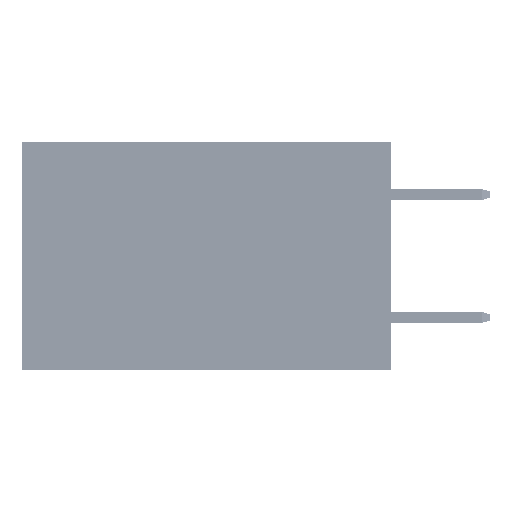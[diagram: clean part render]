
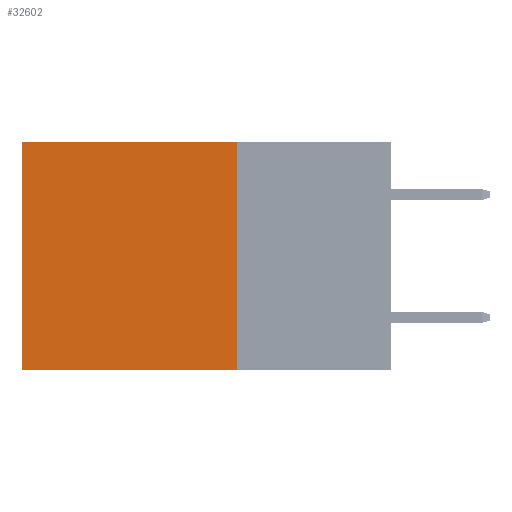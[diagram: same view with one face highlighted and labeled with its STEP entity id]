
A CAD part, left-side view. The second image highlights one B-rep face of the part: STEP entity #32602.
In plain terms, the highlighted planar face has unit normal (-1, 0, 0).
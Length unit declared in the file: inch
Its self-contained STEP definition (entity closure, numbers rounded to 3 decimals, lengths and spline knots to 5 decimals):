
#63 = DIRECTION ( 'NONE',  ( 0., 1., 0. ) ) ;
#660 = LINE ( 'NONE', #8507, #33065 ) ;
#1041 = CARTESIAN_POINT ( 'NONE',  ( 0.2875, 0.25, 0. ) ) ;
#6614 = LINE ( 'NONE', #29892, #17607 ) ;
#6809 = DIRECTION ( 'NONE',  ( 0., 0., -1. ) ) ;
#6989 = FACE_OUTER_BOUND ( 'NONE', #10618, .T. ) ;
#7064 = CARTESIAN_POINT ( 'NONE',  ( 0.2875, 0.6, 0. ) ) ;
#7995 = ORIENTED_EDGE ( 'NONE', *, *, #26236, .F. ) ;
#8343 = DIRECTION ( 'NONE',  ( 0., 0., -1. ) ) ;
#8507 = CARTESIAN_POINT ( 'NONE',  ( 0.2875, 0.25, 0. ) ) ;
#8690 = VECTOR ( 'NONE', #63, 39.37008 ) ;
#10618 = EDGE_LOOP ( 'NONE', ( #33164, #28526, #7995, #21741 ) ) ;
#11843 = CARTESIAN_POINT ( 'NONE',  ( 0.2875, 0.25, -0.37 ) ) ;
#12913 = AXIS2_PLACEMENT_3D ( 'NONE', #33566, #41643, #41468 ) ;
#14683 = VERTEX_POINT ( 'NONE', #1041 ) ;
#16179 = CARTESIAN_POINT ( 'NONE',  ( 0.2875, 0.25, -0.37 ) ) ;
#17534 = DIRECTION ( 'NONE',  ( 0., 1., 0. ) ) ;
#17607 = VECTOR ( 'NONE', #6809, 39.37008 ) ;
#17733 = EDGE_CURVE ( 'NONE', #26829, #38961, #19094, .T. ) ;
#19071 = VECTOR ( 'NONE', #17534, 39.37008 ) ;
#19094 = LINE ( 'NONE', #11843, #8690 ) ;
#21741 = ORIENTED_EDGE ( 'NONE', *, *, #33916, .T. ) ;
#25809 = LINE ( 'NONE', #36885, #19071 ) ;
#26236 = EDGE_CURVE ( 'NONE', #14683, #26829, #660, .T. ) ;
#26829 = VERTEX_POINT ( 'NONE', #16179 ) ;
#28526 = ORIENTED_EDGE ( 'NONE', *, *, #17733, .F. ) ;
#29892 = CARTESIAN_POINT ( 'NONE',  ( 0.2875, 0.6, 0. ) ) ;
#32602 = ADVANCED_FACE ( 'NONE', ( #6989 ), #37214, .F. ) ;
#33065 = VECTOR ( 'NONE', #8343, 39.37008 ) ;
#33164 = ORIENTED_EDGE ( 'NONE', *, *, #40002, .T. ) ;
#33566 = CARTESIAN_POINT ( 'NONE',  ( 0.2875, 0.25, 0. ) ) ;
#33916 = EDGE_CURVE ( 'NONE', #14683, #39538, #25809, .T. ) ;
#34966 = CARTESIAN_POINT ( 'NONE',  ( 0.2875, 0.6, -0.37 ) ) ;
#36885 = CARTESIAN_POINT ( 'NONE',  ( 0.2875, 0.25, 0. ) ) ;
#37214 = PLANE ( 'NONE',  #12913 ) ;
#38961 = VERTEX_POINT ( 'NONE', #34966 ) ;
#39538 = VERTEX_POINT ( 'NONE', #7064 ) ;
#40002 = EDGE_CURVE ( 'NONE', #39538, #38961, #6614, .T. ) ;
#41468 = DIRECTION ( 'NONE',  ( 0., 0., -1. ) ) ;
#41643 = DIRECTION ( 'NONE',  ( 1., 0., 0. ) ) ;
